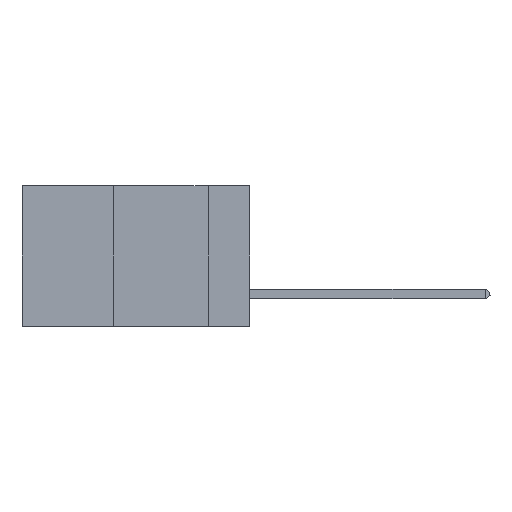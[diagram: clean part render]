
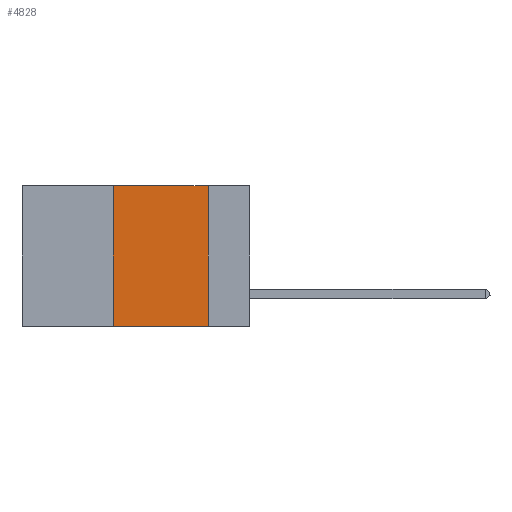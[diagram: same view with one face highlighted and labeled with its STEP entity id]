
A CAD part, left-side view. The second image highlights one B-rep face of the part: STEP entity #4828.
In plain terms, the highlighted planar face has unit normal (-1, 0, 0).
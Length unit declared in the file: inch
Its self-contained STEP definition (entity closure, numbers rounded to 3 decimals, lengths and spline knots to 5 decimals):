
#140 = VERTEX_POINT ( 'NONE', #6526 ) ;
#258 = DIRECTION ( 'NONE',  ( 0., -1., 0. ) ) ;
#671 = VECTOR ( 'NONE', #7034, 39.37008 ) ;
#1429 = VECTOR ( 'NONE', #12840, 39.37008 ) ;
#2134 = DIRECTION ( 'NONE',  ( 1., 0., 0. ) ) ;
#2252 = CARTESIAN_POINT ( 'NONE',  ( 0., 0.6, 0. ) ) ;
#2740 = LINE ( 'NONE', #14930, #671 ) ;
#2753 = CARTESIAN_POINT ( 'NONE',  ( 0., 0.36, -0.37 ) ) ;
#2881 = LINE ( 'NONE', #16654, #1429 ) ;
#2968 = FACE_OUTER_BOUND ( 'NONE', #3609, .T. ) ;
#3090 = LINE ( 'NONE', #7796, #16514 ) ;
#3609 = EDGE_LOOP ( 'NONE', ( #5139, #7490, #14825, #5882 ) ) ;
#4301 = VERTEX_POINT ( 'NONE', #7395 ) ;
#4828 = ADVANCED_FACE ( 'NONE', ( #2968 ), #14287, .F. ) ;
#4966 = VERTEX_POINT ( 'NONE', #2753 ) ;
#5139 = ORIENTED_EDGE ( 'NONE', *, *, #13656, .F. ) ;
#5882 = ORIENTED_EDGE ( 'NONE', *, *, #7849, .T. ) ;
#6526 = CARTESIAN_POINT ( 'NONE',  ( 0., 0.11, -0.37 ) ) ;
#7034 = DIRECTION ( 'NONE',  ( 0., 0., -1. ) ) ;
#7259 = LINE ( 'NONE', #7995, #11582 ) ;
#7395 = CARTESIAN_POINT ( 'NONE',  ( 0., 0.11, 0. ) ) ;
#7490 = ORIENTED_EDGE ( 'NONE', *, *, #9266, .F. ) ;
#7796 = CARTESIAN_POINT ( 'NONE',  ( 0., 0.6, -0.37 ) ) ;
#7849 = EDGE_CURVE ( 'NONE', #4966, #140, #3090, .T. ) ;
#7995 = CARTESIAN_POINT ( 'NONE',  ( 0., 0.6, 0. ) ) ;
#9266 = EDGE_CURVE ( 'NONE', #12186, #4301, #7259, .T. ) ;
#9509 = EDGE_CURVE ( 'NONE', #4966, #12186, #2881, .T. ) ;
#9944 = AXIS2_PLACEMENT_3D ( 'NONE', #2252, #2134, #15097 ) ;
#11582 = VECTOR ( 'NONE', #258, 39.37008 ) ;
#12186 = VERTEX_POINT ( 'NONE', #14761 ) ;
#12786 = DIRECTION ( 'NONE',  ( 0., -1., 0. ) ) ;
#12840 = DIRECTION ( 'NONE',  ( 0., 0., 1. ) ) ;
#13656 = EDGE_CURVE ( 'NONE', #4301, #140, #2740, .T. ) ;
#14287 = PLANE ( 'NONE',  #9944 ) ;
#14761 = CARTESIAN_POINT ( 'NONE',  ( 0., 0.36, 0. ) ) ;
#14825 = ORIENTED_EDGE ( 'NONE', *, *, #9509, .F. ) ;
#14930 = CARTESIAN_POINT ( 'NONE',  ( 0., 0.11, 0. ) ) ;
#15097 = DIRECTION ( 'NONE',  ( 0., 0., -1. ) ) ;
#16514 = VECTOR ( 'NONE', #12786, 39.37008 ) ;
#16654 = CARTESIAN_POINT ( 'NONE',  ( 0., 0.36, 0. ) ) ;
